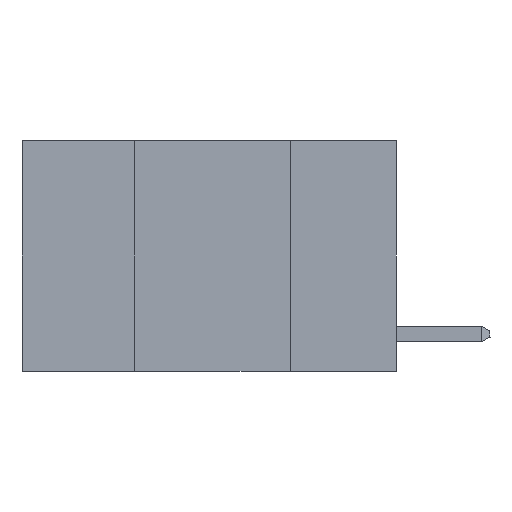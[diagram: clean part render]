
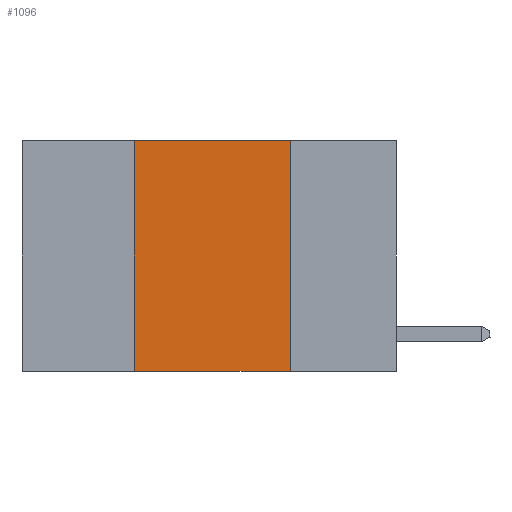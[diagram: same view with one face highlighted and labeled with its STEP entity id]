
A CAD part, left-side view. The second image highlights one B-rep face of the part: STEP entity #1096.
In plain terms, the highlighted planar face has unit normal (-1, 0, 0).
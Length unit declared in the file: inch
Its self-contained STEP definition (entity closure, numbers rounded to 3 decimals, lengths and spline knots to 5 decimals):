
#629 = VERTEX_POINT ( 'NONE', #3836 ) ;
#821 = AXIS2_PLACEMENT_3D ( 'NONE', #10555, #13148, #13770 ) ;
#1096 = ADVANCED_FACE ( 'NONE', ( #17295 ), #8916, .F. ) ;
#1155 = CARTESIAN_POINT ( 'NONE',  ( 0., 0.17, -0.37 ) ) ;
#1201 = DIRECTION ( 'NONE',  ( 0., -1., 0. ) ) ;
#1568 = LINE ( 'NONE', #16956, #8340 ) ;
#2797 = ORIENTED_EDGE ( 'NONE', *, *, #15815, .F. ) ;
#3836 = CARTESIAN_POINT ( 'NONE',  ( 0., 0.42, 0. ) ) ;
#4204 = VERTEX_POINT ( 'NONE', #5171 ) ;
#5171 = CARTESIAN_POINT ( 'NONE',  ( 0., 0.17, 0. ) ) ;
#5987 = CARTESIAN_POINT ( 'NONE',  ( 0., 0.17, 0. ) ) ;
#7823 = CARTESIAN_POINT ( 'NONE',  ( 0., 0.42, -0.37 ) ) ;
#7830 = LINE ( 'NONE', #5987, #11839 ) ;
#8340 = VECTOR ( 'NONE', #9596, 39.37008 ) ;
#8460 = EDGE_LOOP ( 'NONE', ( #10029, #13995, #2797, #18294 ) ) ;
#8792 = VERTEX_POINT ( 'NONE', #7823 ) ;
#8916 = PLANE ( 'NONE',  #821 ) ;
#9500 = VECTOR ( 'NONE', #1201, 39.37008 ) ;
#9596 = DIRECTION ( 'NONE',  ( 0., -1., 0. ) ) ;
#10029 = ORIENTED_EDGE ( 'NONE', *, *, #13843, .F. ) ;
#10555 = CARTESIAN_POINT ( 'NONE',  ( 0., 0.6, 0. ) ) ;
#11025 = VECTOR ( 'NONE', #13349, 39.37008 ) ;
#11839 = VECTOR ( 'NONE', #14818, 39.37008 ) ;
#12393 = VERTEX_POINT ( 'NONE', #1155 ) ;
#13148 = DIRECTION ( 'NONE',  ( 1., 0., 0. ) ) ;
#13349 = DIRECTION ( 'NONE',  ( 0., 0., 1. ) ) ;
#13770 = DIRECTION ( 'NONE',  ( 0., 0., -1. ) ) ;
#13843 = EDGE_CURVE ( 'NONE', #4204, #12393, #7830, .T. ) ;
#13995 = ORIENTED_EDGE ( 'NONE', *, *, #18839, .F. ) ;
#14818 = DIRECTION ( 'NONE',  ( 0., 0., -1. ) ) ;
#15815 = EDGE_CURVE ( 'NONE', #8792, #629, #18797, .T. ) ;
#16956 = CARTESIAN_POINT ( 'NONE',  ( 0., 0.6, -0.37 ) ) ;
#17254 = CARTESIAN_POINT ( 'NONE',  ( 0., 0.6, 0. ) ) ;
#17295 = FACE_OUTER_BOUND ( 'NONE', #8460, .T. ) ;
#17334 = LINE ( 'NONE', #17254, #9500 ) ;
#17706 = CARTESIAN_POINT ( 'NONE',  ( 0., 0.42, 0. ) ) ;
#18294 = ORIENTED_EDGE ( 'NONE', *, *, #18704, .T. ) ;
#18704 = EDGE_CURVE ( 'NONE', #8792, #12393, #1568, .T. ) ;
#18797 = LINE ( 'NONE', #17706, #11025 ) ;
#18839 = EDGE_CURVE ( 'NONE', #629, #4204, #17334, .T. ) ;
